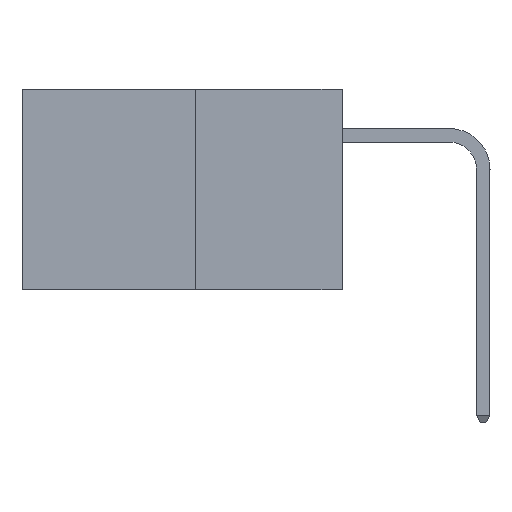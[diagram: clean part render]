
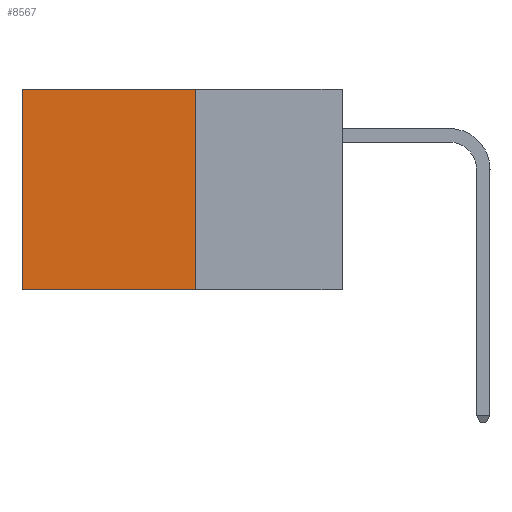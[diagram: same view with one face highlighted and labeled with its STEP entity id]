
A CAD part, left-side view. The second image highlights one B-rep face of the part: STEP entity #8567.
In plain terms, the highlighted planar face has unit normal (-1, 0, 0).
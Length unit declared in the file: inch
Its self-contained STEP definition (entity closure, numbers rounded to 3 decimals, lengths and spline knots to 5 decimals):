
#334 = VERTEX_POINT ( 'NONE', #2664 ) ;
#599 = VECTOR ( 'NONE', #7854, 39.37008 ) ;
#872 = CARTESIAN_POINT ( 'NONE',  ( 0.277, 0.27, 0. ) ) ;
#933 = DIRECTION ( 'NONE',  ( 0., 1., 0. ) ) ;
#1469 = FACE_OUTER_BOUND ( 'NONE', #9611, .T. ) ;
#1592 = CARTESIAN_POINT ( 'NONE',  ( 0.277, 0.27, 0. ) ) ;
#1698 = VECTOR ( 'NONE', #933, 39.37008 ) ;
#1971 = PLANE ( 'NONE',  #7445 ) ;
#2211 = ORIENTED_EDGE ( 'NONE', *, *, #8597, .T. ) ;
#2263 = ORIENTED_EDGE ( 'NONE', *, *, #8662, .F. ) ;
#2288 = VERTEX_POINT ( 'NONE', #4042 ) ;
#2334 = ORIENTED_EDGE ( 'NONE', *, *, #3257, .F. ) ;
#2345 = ORIENTED_EDGE ( 'NONE', *, *, #3060, .T. ) ;
#2664 = CARTESIAN_POINT ( 'NONE',  ( 0.277, 0.27, -0.37 ) ) ;
#3060 = EDGE_CURVE ( 'NONE', #7929, #2288, #8233, .T. ) ;
#3257 = EDGE_CURVE ( 'NONE', #7929, #334, #10424, .T. ) ;
#3819 = CARTESIAN_POINT ( 'NONE',  ( 0.277, 0.27, -0.37 ) ) ;
#4042 = CARTESIAN_POINT ( 'NONE',  ( 0.277, 0.59, 0. ) ) ;
#4566 = CARTESIAN_POINT ( 'NONE',  ( 0.277, 0.27, -0.37 ) ) ;
#5253 = VERTEX_POINT ( 'NONE', #7280 ) ;
#5408 = DIRECTION ( 'NONE',  ( 0., 0., -1. ) ) ;
#6243 = CARTESIAN_POINT ( 'NONE',  ( 0.277, 0.59, -0.37 ) ) ;
#7156 = LINE ( 'NONE', #3819, #599 ) ;
#7280 = CARTESIAN_POINT ( 'NONE',  ( 0.277, 0.59, -0.37 ) ) ;
#7445 = AXIS2_PLACEMENT_3D ( 'NONE', #4566, #9880, #5408 ) ;
#7854 = DIRECTION ( 'NONE',  ( 0., 1., 0. ) ) ;
#7929 = VERTEX_POINT ( 'NONE', #1592 ) ;
#8063 = DIRECTION ( 'NONE',  ( 0., 0., -1. ) ) ;
#8233 = LINE ( 'NONE', #872, #1698 ) ;
#8304 = CARTESIAN_POINT ( 'NONE',  ( 0.277, 0.27, -0.37 ) ) ;
#8338 = VECTOR ( 'NONE', #8063, 39.37008 ) ;
#8567 = ADVANCED_FACE ( 'NONE', ( #1469 ), #1971, .F. ) ;
#8597 = EDGE_CURVE ( 'NONE', #2288, #5253, #10155, .T. ) ;
#8662 = EDGE_CURVE ( 'NONE', #334, #5253, #7156, .T. ) ;
#9492 = VECTOR ( 'NONE', #9913, 39.37008 ) ;
#9611 = EDGE_LOOP ( 'NONE', ( #2211, #2263, #2334, #2345 ) ) ;
#9880 = DIRECTION ( 'NONE',  ( 1., 0., 0. ) ) ;
#9913 = DIRECTION ( 'NONE',  ( 0., 0., -1. ) ) ;
#10155 = LINE ( 'NONE', #6243, #9492 ) ;
#10424 = LINE ( 'NONE', #8304, #8338 ) ;
